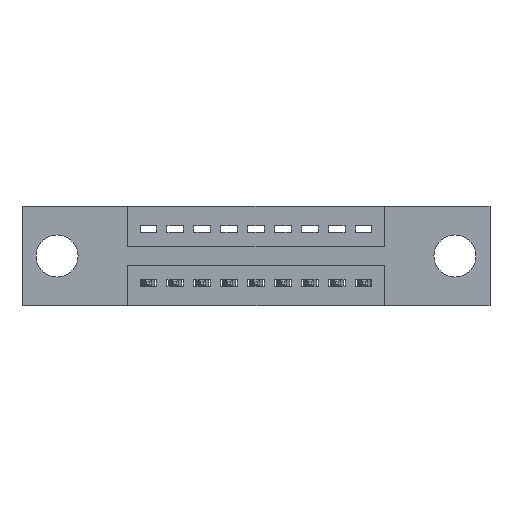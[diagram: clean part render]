
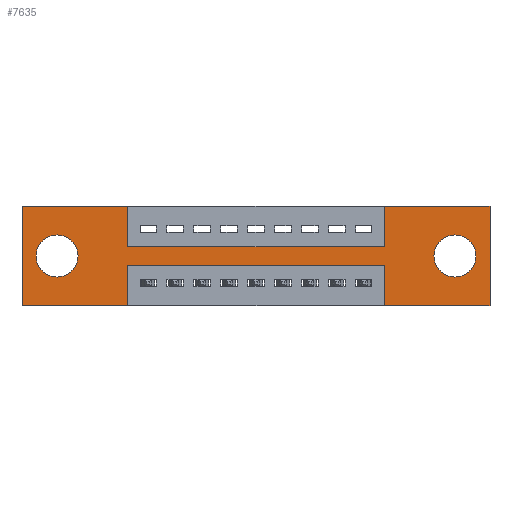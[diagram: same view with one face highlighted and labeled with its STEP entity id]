
A CAD part, front view. The second image highlights one B-rep face of the part: STEP entity #7635.
In plain terms, the highlighted planar face has unit normal (0, -1, 0).
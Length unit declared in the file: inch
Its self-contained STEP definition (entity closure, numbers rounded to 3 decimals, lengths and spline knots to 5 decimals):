
#82 = VERTEX_POINT ( 'NONE', #3108 ) ;
#619 = CARTESIAN_POINT ( 'NONE',  ( 0., 0., 0. ) ) ;
#735 = EDGE_CURVE ( 'NONE', #7110, #883, #2515, .T. ) ;
#763 = ORIENTED_EDGE ( 'NONE', *, *, #9241, .T. ) ;
#769 = CARTESIAN_POINT ( 'NONE',  ( 0., 0., 0. ) ) ;
#776 = ORIENTED_EDGE ( 'NONE', *, *, #9059, .T. ) ;
#852 = ORIENTED_EDGE ( 'NONE', *, *, #905, .T. ) ;
#883 = VERTEX_POINT ( 'NONE', #6545 ) ;
#905 = EDGE_CURVE ( 'NONE', #82, #4928, #5043, .T. ) ;
#1051 = VERTEX_POINT ( 'NONE', #11148 ) ;
#1221 = VECTOR ( 'NONE', #9170, 39.37008 ) ;
#1285 = CARTESIAN_POINT ( 'NONE',  ( 0., 0., -0.37 ) ) ;
#1430 = VECTOR ( 'NONE', #3559, 39.37008 ) ;
#1480 = EDGE_CURVE ( 'NONE', #3495, #10323, #3673, .T. ) ;
#1621 = CARTESIAN_POINT ( 'NONE',  ( 1.735, 0., 0. ) ) ;
#1662 = AXIS2_PLACEMENT_3D ( 'NONE', #6018, #10911, #6390 ) ;
#1700 = VERTEX_POINT ( 'NONE', #4922 ) ;
#1734 = DIRECTION ( 'NONE',  ( 1., 0., 0. ) ) ;
#1761 = EDGE_LOOP ( 'NONE', ( #763, #2638 ) ) ;
#1788 = DIRECTION ( 'NONE',  ( 0., 0., 1. ) ) ;
#1845 = VECTOR ( 'NONE', #10035, 39.37008 ) ;
#1848 = CARTESIAN_POINT ( 'NONE',  ( 1.3425, 0., 0. ) ) ;
#1875 = ORIENTED_EDGE ( 'NONE', *, *, #5733, .F. ) ;
#1947 = DIRECTION ( 'NONE',  ( 0., 0., -1. ) ) ;
#2027 = DIRECTION ( 'NONE',  ( -1., 0., 0. ) ) ;
#2094 = VECTOR ( 'NONE', #8040, 39.37008 ) ;
#2117 = ORIENTED_EDGE ( 'NONE', *, *, #2610, .F. ) ;
#2166 = CIRCLE ( 'NONE', #7924, 0.078 ) ;
#2331 = LINE ( 'NONE', #9623, #10786 ) ;
#2393 = LINE ( 'NONE', #10062, #1845 ) ;
#2426 = VECTOR ( 'NONE', #2027, 39.37008 ) ;
#2498 = VERTEX_POINT ( 'NONE', #9790 ) ;
#2515 = LINE ( 'NONE', #7060, #9051 ) ;
#2610 = EDGE_CURVE ( 'NONE', #883, #7677, #2777, .T. ) ;
#2635 = ORIENTED_EDGE ( 'NONE', *, *, #6143, .F. ) ;
#2638 = ORIENTED_EDGE ( 'NONE', *, *, #9927, .T. ) ;
#2774 = AXIS2_PLACEMENT_3D ( 'NONE', #10015, #5115, #10843 ) ;
#2777 = LINE ( 'NONE', #10862, #7095 ) ;
#2800 = ORIENTED_EDGE ( 'NONE', *, *, #9235, .F. ) ;
#2992 = EDGE_CURVE ( 'NONE', #2498, #3828, #7843, .T. ) ;
#3105 = ORIENTED_EDGE ( 'NONE', *, *, #10432, .F. ) ;
#3108 = CARTESIAN_POINT ( 'NONE',  ( 1.605, 0., -0.107 ) ) ;
#3154 = ORIENTED_EDGE ( 'NONE', *, *, #10094, .F. ) ;
#3184 = DIRECTION ( 'NONE',  ( -1., 0., 0. ) ) ;
#3225 = CARTESIAN_POINT ( 'NONE',  ( 0.3925, 0., -0.22 ) ) ;
#3343 = ORIENTED_EDGE ( 'NONE', *, *, #2992, .F. ) ;
#3479 = ORIENTED_EDGE ( 'NONE', *, *, #5942, .F. ) ;
#3495 = VERTEX_POINT ( 'NONE', #9001 ) ;
#3559 = DIRECTION ( 'NONE',  ( 0., 0., -1. ) ) ;
#3633 = EDGE_LOOP ( 'NONE', ( #852, #776 ) ) ;
#3673 = LINE ( 'NONE', #619, #1221 ) ;
#3786 = ORIENTED_EDGE ( 'NONE', *, *, #8124, .F. ) ;
#3828 = VERTEX_POINT ( 'NONE', #6089 ) ;
#3859 = VERTEX_POINT ( 'NONE', #5014 ) ;
#3904 = ORIENTED_EDGE ( 'NONE', *, *, #735, .F. ) ;
#4045 = VERTEX_POINT ( 'NONE', #10149 ) ;
#4060 = PLANE ( 'NONE',  #10925 ) ;
#4166 = AXIS2_PLACEMENT_3D ( 'NONE', #4552, #10270, #5403 ) ;
#4194 = CIRCLE ( 'NONE', #2774, 0.078 ) ;
#4488 = DIRECTION ( 'NONE',  ( 0., 1., 0. ) ) ;
#4552 = CARTESIAN_POINT ( 'NONE',  ( 0.13, 0., -0.185 ) ) ;
#4680 = CARTESIAN_POINT ( 'NONE',  ( 0., 0., -0.37 ) ) ;
#4778 = VECTOR ( 'NONE', #1788, 39.37008 ) ;
#4788 = LINE ( 'NONE', #4680, #2094 ) ;
#4822 = EDGE_CURVE ( 'NONE', #10323, #7110, #2393, .T. ) ;
#4901 = DIRECTION ( 'NONE',  ( 0., 0., -1. ) ) ;
#4907 = LINE ( 'NONE', #3225, #11209 ) ;
#4922 = CARTESIAN_POINT ( 'NONE',  ( 0.3925, 0., -0.22 ) ) ;
#4928 = VERTEX_POINT ( 'NONE', #9409 ) ;
#5014 = CARTESIAN_POINT ( 'NONE',  ( 1.735, 0., -0.37 ) ) ;
#5043 = CIRCLE ( 'NONE', #1662, 0.078 ) ;
#5115 = DIRECTION ( 'NONE',  ( 0., 1., 0. ) ) ;
#5208 = CARTESIAN_POINT ( 'NONE',  ( 0., 0., 0. ) ) ;
#5303 = FACE_BOUND ( 'NONE', #1761, .T. ) ;
#5403 = DIRECTION ( 'NONE',  ( 0., 0., 1. ) ) ;
#5606 = CARTESIAN_POINT ( 'NONE',  ( 0.13, 0., -0.263 ) ) ;
#5654 = EDGE_LOOP ( 'NONE', ( #3786, #3479, #3343, #3154, #3105, #2800, #2635, #2117, #3904, #10219, #7308, #1875 ) ) ;
#5733 = EDGE_CURVE ( 'NONE', #4045, #3495, #4788, .T. ) ;
#5942 = EDGE_CURVE ( 'NONE', #3828, #1700, #4907, .T. ) ;
#6018 = CARTESIAN_POINT ( 'NONE',  ( 1.605, 0., -0.185 ) ) ;
#6089 = CARTESIAN_POINT ( 'NONE',  ( 1.3425, 0., -0.22 ) ) ;
#6143 = EDGE_CURVE ( 'NONE', #7677, #6705, #6995, .T. ) ;
#6151 = CARTESIAN_POINT ( 'NONE',  ( 1.735, 0., 0. ) ) ;
#6390 = DIRECTION ( 'NONE',  ( 0., 0., -1. ) ) ;
#6545 = CARTESIAN_POINT ( 'NONE',  ( 0.3925, 0., -0.15 ) ) ;
#6705 = VERTEX_POINT ( 'NONE', #8661 ) ;
#6710 = VECTOR ( 'NONE', #7145, 39.37008 ) ;
#6752 = CARTESIAN_POINT ( 'NONE',  ( 0.3925, 0., 0. ) ) ;
#6995 = LINE ( 'NONE', #1848, #4778 ) ;
#7060 = CARTESIAN_POINT ( 'NONE',  ( 0.3925, 0., 0. ) ) ;
#7095 = VECTOR ( 'NONE', #8433, 39.37008 ) ;
#7110 = VERTEX_POINT ( 'NONE', #6752 ) ;
#7145 = DIRECTION ( 'NONE',  ( 0., 0., 1. ) ) ;
#7198 = VERTEX_POINT ( 'NONE', #1621 ) ;
#7308 = ORIENTED_EDGE ( 'NONE', *, *, #1480, .F. ) ;
#7432 = CARTESIAN_POINT ( 'NONE',  ( 1.3425, 0., -0.37 ) ) ;
#7448 = CARTESIAN_POINT ( 'NONE',  ( 1.3425, 0., -0.15 ) ) ;
#7495 = FACE_OUTER_BOUND ( 'NONE', #5654, .T. ) ;
#7635 = ADVANCED_FACE ( 'NONE', ( #9413, #5303, #7495 ), #4060, .T. ) ;
#7677 = VERTEX_POINT ( 'NONE', #7448 ) ;
#7843 = LINE ( 'NONE', #7432, #6710 ) ;
#7924 = AXIS2_PLACEMENT_3D ( 'NONE', #9426, #4488, #10207 ) ;
#8040 = DIRECTION ( 'NONE',  ( -1., 0., 0. ) ) ;
#8043 = CARTESIAN_POINT ( 'NONE',  ( 0., 0., -0.37 ) ) ;
#8124 = EDGE_CURVE ( 'NONE', #1700, #4045, #2331, .T. ) ;
#8188 = VERTEX_POINT ( 'NONE', #5606 ) ;
#8333 = CIRCLE ( 'NONE', #4166, 0.078 ) ;
#8433 = DIRECTION ( 'NONE',  ( 1., 0., 0. ) ) ;
#8661 = CARTESIAN_POINT ( 'NONE',  ( 1.3425, 0., 0. ) ) ;
#8719 = LINE ( 'NONE', #8043, #2426 ) ;
#8993 = VECTOR ( 'NONE', #1734, 39.37008 ) ;
#9001 = CARTESIAN_POINT ( 'NONE',  ( 0., 0., -0.37 ) ) ;
#9051 = VECTOR ( 'NONE', #9521, 39.37008 ) ;
#9059 = EDGE_CURVE ( 'NONE', #4928, #82, #4194, .T. ) ;
#9170 = DIRECTION ( 'NONE',  ( 0., 0., 1. ) ) ;
#9235 = EDGE_CURVE ( 'NONE', #6705, #7198, #11154, .T. ) ;
#9241 = EDGE_CURVE ( 'NONE', #1051, #8188, #2166, .T. ) ;
#9409 = CARTESIAN_POINT ( 'NONE',  ( 1.605, 0., -0.263 ) ) ;
#9413 = FACE_BOUND ( 'NONE', #3633, .T. ) ;
#9426 = CARTESIAN_POINT ( 'NONE',  ( 0.13, 0., -0.185 ) ) ;
#9521 = DIRECTION ( 'NONE',  ( 0., 0., -1. ) ) ;
#9623 = CARTESIAN_POINT ( 'NONE',  ( 0.3925, 0., -0.37 ) ) ;
#9722 = LINE ( 'NONE', #6151, #1430 ) ;
#9790 = CARTESIAN_POINT ( 'NONE',  ( 1.3425, 0., -0.37 ) ) ;
#9831 = DIRECTION ( 'NONE',  ( 0., -1., 0. ) ) ;
#9927 = EDGE_CURVE ( 'NONE', #8188, #1051, #8333, .T. ) ;
#10015 = CARTESIAN_POINT ( 'NONE',  ( 1.605, 0., -0.185 ) ) ;
#10035 = DIRECTION ( 'NONE',  ( 1., 0., 0. ) ) ;
#10062 = CARTESIAN_POINT ( 'NONE',  ( 0., 0., 0. ) ) ;
#10094 = EDGE_CURVE ( 'NONE', #3859, #2498, #8719, .T. ) ;
#10149 = CARTESIAN_POINT ( 'NONE',  ( 0.3925, 0., -0.37 ) ) ;
#10207 = DIRECTION ( 'NONE',  ( 0., 0., 1. ) ) ;
#10219 = ORIENTED_EDGE ( 'NONE', *, *, #4822, .F. ) ;
#10270 = DIRECTION ( 'NONE',  ( 0., 1., 0. ) ) ;
#10323 = VERTEX_POINT ( 'NONE', #5208 ) ;
#10432 = EDGE_CURVE ( 'NONE', #7198, #3859, #9722, .T. ) ;
#10786 = VECTOR ( 'NONE', #1947, 39.37008 ) ;
#10843 = DIRECTION ( 'NONE',  ( 0., 0., -1. ) ) ;
#10862 = CARTESIAN_POINT ( 'NONE',  ( 0.3925, 0., -0.15 ) ) ;
#10911 = DIRECTION ( 'NONE',  ( 0., 1., 0. ) ) ;
#10925 = AXIS2_PLACEMENT_3D ( 'NONE', #1285, #9831, #4901 ) ;
#11148 = CARTESIAN_POINT ( 'NONE',  ( 0.13, 0., -0.107 ) ) ;
#11154 = LINE ( 'NONE', #769, #8993 ) ;
#11209 = VECTOR ( 'NONE', #3184, 39.37008 ) ;
